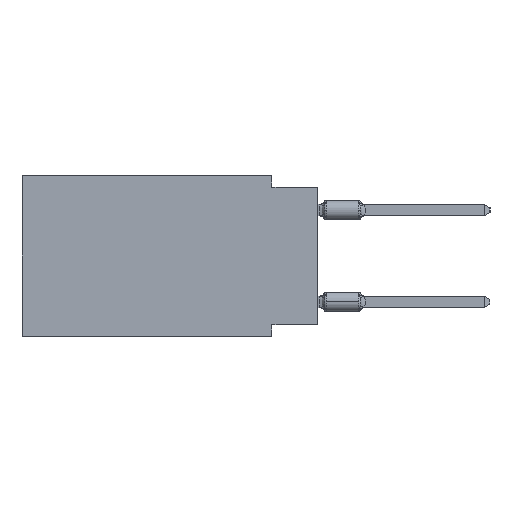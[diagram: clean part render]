
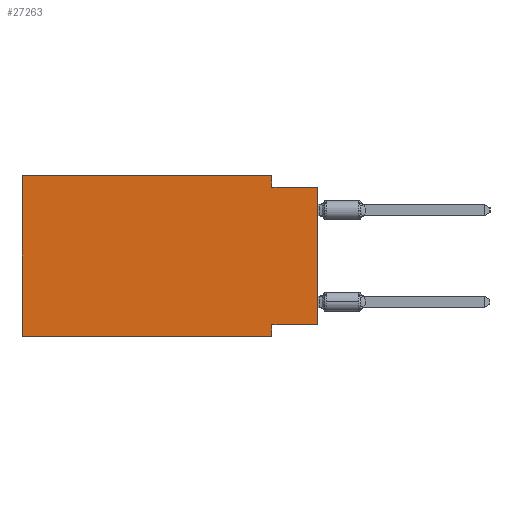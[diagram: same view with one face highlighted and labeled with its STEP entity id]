
A CAD part, left-side view. The second image highlights one B-rep face of the part: STEP entity #27263.
In plain terms, the highlighted planar face has unit normal (-1, 0, 0).
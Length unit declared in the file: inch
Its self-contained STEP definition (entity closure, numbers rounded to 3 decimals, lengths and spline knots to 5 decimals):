
#393 = VERTEX_POINT ( 'NONE', #16682 ) ;
#406 = ORIENTED_EDGE ( 'NONE', *, *, #2503, .F. ) ;
#583 = VERTEX_POINT ( 'NONE', #10359 ) ;
#1602 = CARTESIAN_POINT ( 'NONE',  ( 0., 0.645, 0. ) ) ;
#2503 = EDGE_CURVE ( 'NONE', #12392, #393, #25282, .T. ) ;
#3215 = EDGE_LOOP ( 'NONE', ( #24543, #6969, #406, #16434, #15820, #7498, #24796, #9396 ) ) ;
#3287 = VERTEX_POINT ( 'NONE', #6755 ) ;
#3628 = CARTESIAN_POINT ( 'NONE',  ( 0., 0.645, 0. ) ) ;
#5107 = CARTESIAN_POINT ( 'NONE',  ( 0., 0.1, -0.35 ) ) ;
#5884 = CARTESIAN_POINT ( 'NONE',  ( 0., 0., -0.325 ) ) ;
#6755 = CARTESIAN_POINT ( 'NONE',  ( 0., 0.645, 0. ) ) ;
#6969 = ORIENTED_EDGE ( 'NONE', *, *, #24160, .F. ) ;
#7498 = ORIENTED_EDGE ( 'NONE', *, *, #16068, .T. ) ;
#9396 = ORIENTED_EDGE ( 'NONE', *, *, #21110, .F. ) ;
#9832 = VECTOR ( 'NONE', #11983, 39.37008 ) ;
#10359 = CARTESIAN_POINT ( 'NONE',  ( 0., 0.1, -0.325 ) ) ;
#10966 = LINE ( 'NONE', #3628, #32328 ) ;
#11308 = DIRECTION ( 'NONE',  ( 0., -1., 0. ) ) ;
#11709 = DIRECTION ( 'NONE',  ( 0., -1., 0. ) ) ;
#11848 = VECTOR ( 'NONE', #13878, 39.37008 ) ;
#11983 = DIRECTION ( 'NONE',  ( 0., 0., 1. ) ) ;
#12392 = VERTEX_POINT ( 'NONE', #27853 ) ;
#13099 = DIRECTION ( 'NONE',  ( 0., 0., -1. ) ) ;
#13336 = VECTOR ( 'NONE', #15267, 39.37008 ) ;
#13617 = CARTESIAN_POINT ( 'NONE',  ( 0., 0.645, 0. ) ) ;
#13878 = DIRECTION ( 'NONE',  ( 0., 1., 0. ) ) ;
#14252 = EDGE_CURVE ( 'NONE', #3287, #12392, #10966, .T. ) ;
#14757 = CARTESIAN_POINT ( 'NONE',  ( 0., 0., 0. ) ) ;
#15267 = DIRECTION ( 'NONE',  ( 0., 0., 1. ) ) ;
#15356 = CARTESIAN_POINT ( 'NONE',  ( 0., 0.645, -0.35 ) ) ;
#15820 = ORIENTED_EDGE ( 'NONE', *, *, #27649, .F. ) ;
#16068 = EDGE_CURVE ( 'NONE', #23834, #29119, #32954, .T. ) ;
#16419 = VERTEX_POINT ( 'NONE', #23754 ) ;
#16434 = ORIENTED_EDGE ( 'NONE', *, *, #14252, .F. ) ;
#16682 = CARTESIAN_POINT ( 'NONE',  ( 0., 0.1, -0.025 ) ) ;
#17276 = DIRECTION ( 'NONE',  ( 0., 0., -1. ) ) ;
#17301 = DIRECTION ( 'NONE',  ( 0., -1., 0. ) ) ;
#17819 = LINE ( 'NONE', #14757, #13336 ) ;
#18022 = CARTESIAN_POINT ( 'NONE',  ( 0., 0., -0.325 ) ) ;
#20224 = LINE ( 'NONE', #5107, #32659 ) ;
#21110 = EDGE_CURVE ( 'NONE', #28291, #583, #26785, .T. ) ;
#21154 = VECTOR ( 'NONE', #11709, 39.37008 ) ;
#22042 = FACE_OUTER_BOUND ( 'NONE', #3215, .T. ) ;
#22278 = AXIS2_PLACEMENT_3D ( 'NONE', #13617, #23468, #17276 ) ;
#22390 = CARTESIAN_POINT ( 'NONE',  ( 0., 0., -0.025 ) ) ;
#23468 = DIRECTION ( 'NONE',  ( 1., 0., 0. ) ) ;
#23754 = CARTESIAN_POINT ( 'NONE',  ( 0., 0., -0.025 ) ) ;
#23834 = VERTEX_POINT ( 'NONE', #15356 ) ;
#24160 = EDGE_CURVE ( 'NONE', #393, #16419, #25107, .T. ) ;
#24543 = ORIENTED_EDGE ( 'NONE', *, *, #31667, .T. ) ;
#24796 = ORIENTED_EDGE ( 'NONE', *, *, #28292, .F. ) ;
#25107 = LINE ( 'NONE', #22390, #21154 ) ;
#25282 = LINE ( 'NONE', #25629, #31871 ) ;
#25629 = CARTESIAN_POINT ( 'NONE',  ( 0., 0.1, 0. ) ) ;
#26785 = LINE ( 'NONE', #5884, #11848 ) ;
#27263 = ADVANCED_FACE ( 'NONE', ( #22042 ), #32438, .F. ) ;
#27649 = EDGE_CURVE ( 'NONE', #23834, #3287, #29849, .T. ) ;
#27853 = CARTESIAN_POINT ( 'NONE',  ( 0., 0.1, 0. ) ) ;
#27885 = VECTOR ( 'NONE', #17301, 39.37008 ) ;
#28291 = VERTEX_POINT ( 'NONE', #18022 ) ;
#28292 = EDGE_CURVE ( 'NONE', #583, #29119, #20224, .T. ) ;
#29119 = VERTEX_POINT ( 'NONE', #33279 ) ;
#29849 = LINE ( 'NONE', #1602, #9832 ) ;
#30069 = DIRECTION ( 'NONE',  ( 0., 0., -1. ) ) ;
#30226 = CARTESIAN_POINT ( 'NONE',  ( 0., 0.645, -0.35 ) ) ;
#31667 = EDGE_CURVE ( 'NONE', #28291, #16419, #17819, .T. ) ;
#31871 = VECTOR ( 'NONE', #30069, 39.37008 ) ;
#32328 = VECTOR ( 'NONE', #11308, 39.37008 ) ;
#32438 = PLANE ( 'NONE',  #22278 ) ;
#32659 = VECTOR ( 'NONE', #13099, 39.37008 ) ;
#32954 = LINE ( 'NONE', #30226, #27885 ) ;
#33279 = CARTESIAN_POINT ( 'NONE',  ( 0., 0.1, -0.35 ) ) ;
